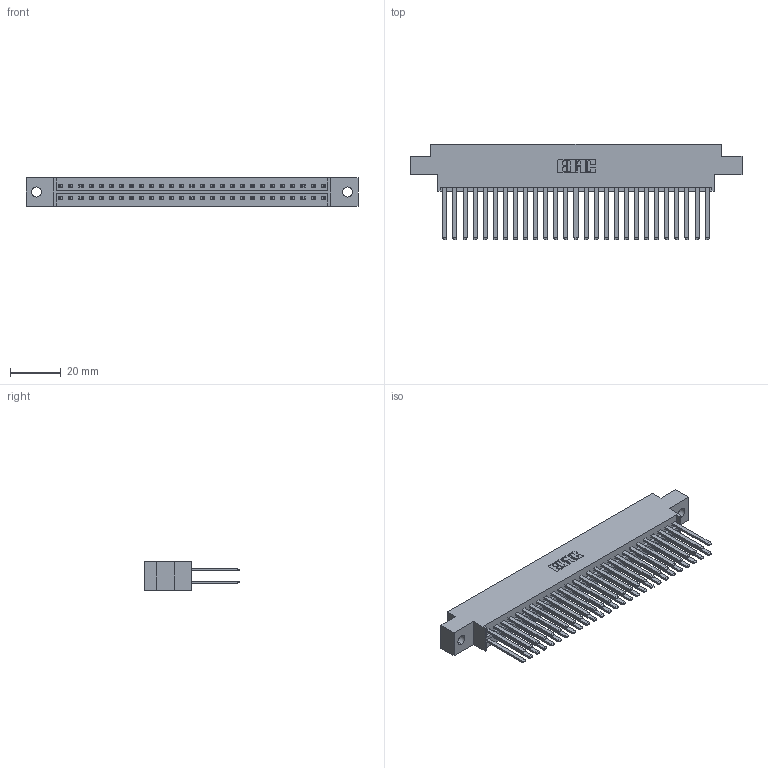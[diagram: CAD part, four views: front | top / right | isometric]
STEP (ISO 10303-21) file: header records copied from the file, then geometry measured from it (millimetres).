
FILE_DESCRIPTION (( 'STEP AP203' ), '1' );
FILE_NAME ('336-054-541-804.STEP', '2020-08-08T00:21:18', ( '' ), ( '' ), 'SwSTEP 2.0', 'SolidWorks 2020', '' );
FILE_SCHEMA (( 'CONFIG_CONTROL_DESIGN' ));
Length unit declared in the file: inch
Products named in the file (3): 336-054-541-804; 336-290-001_336-290-541; 336 Part_Offset - .156 Dia - TH
Assembly tree (55 placements, depth 2):
  336-054-541-804
    336 Part_Offset - .156 Dia - TH
    336-290-001_336-290-541  x54
Bounding box: 130.38 x 37.34 x 11.1 mm (x, y, z)
Volume: 19569.2 mm3; surface area: 24632.5 mm2
Topology: 55 solids, 55 shells, 2386 faces, 7181 edges, 4750 vertices
Faces by surface type: plane 1478, cylinder 908
Entity records: 22728 total; most frequent: CARTESIAN_POINT 3925, ORIENTED_EDGE 3762, DIRECTION 3269, EDGE_CURVE 1881, LINE 1749, VECTOR 1749, VERTEX_POINT 1252, AXIS2_PLACEMENT_3D 760
